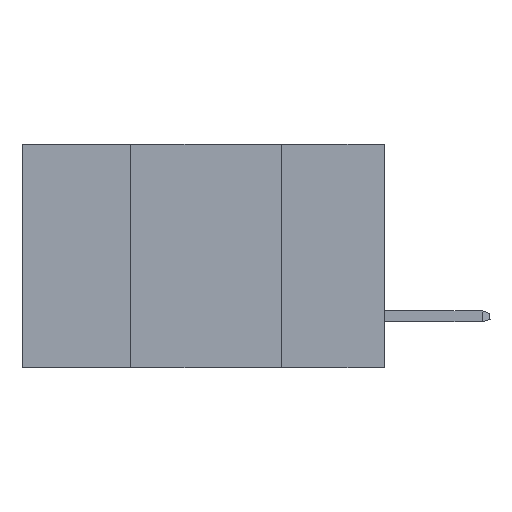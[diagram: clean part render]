
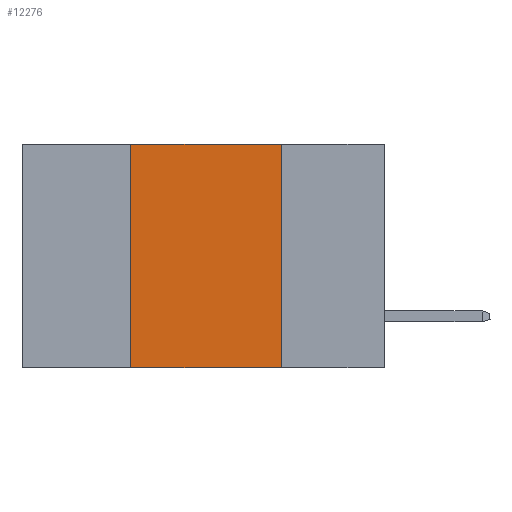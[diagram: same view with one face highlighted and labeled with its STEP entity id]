
A CAD part, left-side view. The second image highlights one B-rep face of the part: STEP entity #12276.
In plain terms, the highlighted planar face has unit normal (-1, 0, 0).
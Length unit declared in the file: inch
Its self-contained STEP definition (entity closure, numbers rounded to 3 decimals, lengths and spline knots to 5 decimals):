
#21 = PLANE ( 'NONE',  #13489 ) ;
#1029 = CARTESIAN_POINT ( 'NONE',  ( 0., 0.6, 0. ) ) ;
#1036 = VERTEX_POINT ( 'NONE', #25643 ) ;
#1363 = CARTESIAN_POINT ( 'NONE',  ( 0., 0.6, -0.37 ) ) ;
#1872 = LINE ( 'NONE', #18535, #23398 ) ;
#1968 = EDGE_CURVE ( 'NONE', #1036, #22318, #1872, .T. ) ;
#2276 = FACE_OUTER_BOUND ( 'NONE', #5068, .T. ) ;
#2660 = EDGE_CURVE ( 'NONE', #21113, #3734, #4878, .T. ) ;
#3650 = CARTESIAN_POINT ( 'NONE',  ( 0., 0.6, 0. ) ) ;
#3734 = VERTEX_POINT ( 'NONE', #16069 ) ;
#4878 = LINE ( 'NONE', #14534, #12441 ) ;
#5068 = EDGE_LOOP ( 'NONE', ( #6501, #19117, #9708, #8424 ) ) ;
#5419 = VECTOR ( 'NONE', #22967, 39.37008 ) ;
#6501 = ORIENTED_EDGE ( 'NONE', *, *, #2660, .F. ) ;
#7567 = DIRECTION ( 'NONE',  ( 0., -1., 0. ) ) ;
#8065 = DIRECTION ( 'NONE',  ( 0., 0., -1. ) ) ;
#8424 = ORIENTED_EDGE ( 'NONE', *, *, #11416, .T. ) ;
#9708 = ORIENTED_EDGE ( 'NONE', *, *, #1968, .F. ) ;
#11416 = EDGE_CURVE ( 'NONE', #1036, #3734, #17418, .T. ) ;
#11880 = LINE ( 'NONE', #1029, #16297 ) ;
#12276 = ADVANCED_FACE ( 'NONE', ( #2276 ), #21, .F. ) ;
#12441 = VECTOR ( 'NONE', #8065, 39.37008 ) ;
#13489 = AXIS2_PLACEMENT_3D ( 'NONE', #3650, #15889, #18172 ) ;
#14534 = CARTESIAN_POINT ( 'NONE',  ( 0., 0.17, 0. ) ) ;
#15889 = DIRECTION ( 'NONE',  ( 1., 0., 0. ) ) ;
#16069 = CARTESIAN_POINT ( 'NONE',  ( 0., 0.17, -0.37 ) ) ;
#16297 = VECTOR ( 'NONE', #7567, 39.37008 ) ;
#17418 = LINE ( 'NONE', #1363, #5419 ) ;
#18172 = DIRECTION ( 'NONE',  ( 0., 0., -1. ) ) ;
#18535 = CARTESIAN_POINT ( 'NONE',  ( 0., 0.42, 0. ) ) ;
#19117 = ORIENTED_EDGE ( 'NONE', *, *, #21594, .F. ) ;
#21113 = VERTEX_POINT ( 'NONE', #22353 ) ;
#21594 = EDGE_CURVE ( 'NONE', #22318, #21113, #11880, .T. ) ;
#21797 = CARTESIAN_POINT ( 'NONE',  ( 0., 0.42, 0. ) ) ;
#22318 = VERTEX_POINT ( 'NONE', #21797 ) ;
#22353 = CARTESIAN_POINT ( 'NONE',  ( 0., 0.17, 0. ) ) ;
#22914 = DIRECTION ( 'NONE',  ( 0., 0., 1. ) ) ;
#22967 = DIRECTION ( 'NONE',  ( 0., -1., 0. ) ) ;
#23398 = VECTOR ( 'NONE', #22914, 39.37008 ) ;
#25643 = CARTESIAN_POINT ( 'NONE',  ( 0., 0.42, -0.37 ) ) ;
